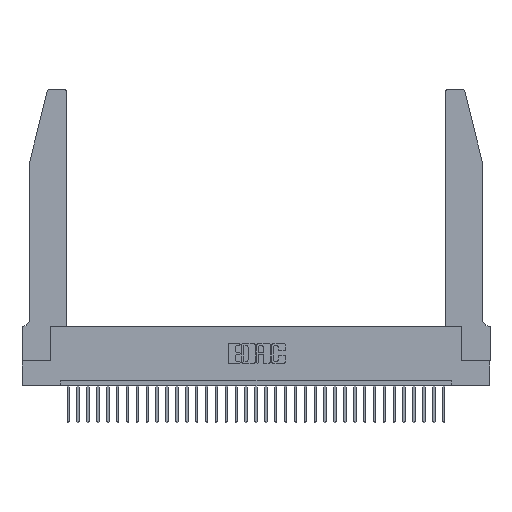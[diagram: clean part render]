
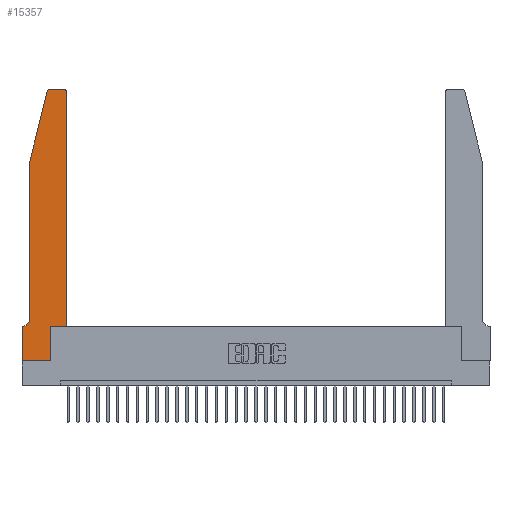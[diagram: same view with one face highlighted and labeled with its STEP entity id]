
A CAD part, top view. The second image highlights one B-rep face of the part: STEP entity #15357.
In plain terms, the highlighted planar face has unit normal (0, 0, 1).
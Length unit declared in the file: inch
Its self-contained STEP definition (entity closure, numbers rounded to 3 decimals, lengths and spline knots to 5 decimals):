
#844 = CARTESIAN_POINT ( 'NONE',  ( 0.0755, 0.42, 0.37 ) ) ;
#1796 = DIRECTION ( 'NONE',  ( -0.239, -0.971, 0. ) ) ;
#1856 = CARTESIAN_POINT ( 'NONE',  ( 0., 0.35, 0.37 ) ) ;
#1897 = ORIENTED_EDGE ( 'NONE', *, *, #27812, .T. ) ;
#1990 = DIRECTION ( 'NONE',  ( 1., 0., 0. ) ) ;
#2243 = EDGE_CURVE ( 'NONE', #21953, #29649, #5907, .T. ) ;
#2429 = LINE ( 'NONE', #12563, #29911 ) ;
#2509 = VERTEX_POINT ( 'NONE', #20249 ) ;
#2885 = CARTESIAN_POINT ( 'NONE',  ( 0., 0., 0.37 ) ) ;
#3509 = DIRECTION ( 'NONE',  ( 1., 0., 0. ) ) ;
#3800 = VECTOR ( 'NONE', #12660, 39.37008 ) ;
#3824 = VERTEX_POINT ( 'NONE', #31055 ) ;
#3830 = ORIENTED_EDGE ( 'NONE', *, *, #16353, .T. ) ;
#4222 = LINE ( 'NONE', #16829, #23867 ) ;
#4612 = AXIS2_PLACEMENT_3D ( 'NONE', #13760, #29898, #32362 ) ;
#4707 = CARTESIAN_POINT ( 'NONE',  ( 0.2865, 0., 0.37 ) ) ;
#4826 = CARTESIAN_POINT ( 'NONE',  ( 0.4505, 2.72, 0.37 ) ) ;
#4992 = EDGE_CURVE ( 'NONE', #17499, #3824, #20780, .T. ) ;
#5145 = EDGE_CURVE ( 'NONE', #8840, #14977, #25309, .T. ) ;
#5199 = LINE ( 'NONE', #14742, #25216 ) ;
#5727 = CARTESIAN_POINT ( 'NONE',  ( 0.0055, 0.35, 0.37 ) ) ;
#5907 = LINE ( 'NONE', #14757, #10103 ) ;
#6216 = LINE ( 'NONE', #22198, #16663 ) ;
#6361 = AXIS2_PLACEMENT_3D ( 'NONE', #10752, #32404, #3509 ) ;
#7086 = EDGE_CURVE ( 'NONE', #14977, #27665, #5199, .T. ) ;
#7990 = LINE ( 'NONE', #28600, #3800 ) ;
#8084 = VERTEX_POINT ( 'NONE', #11076 ) ;
#8706 = CARTESIAN_POINT ( 'NONE',  ( 0.4505, 0.35, 0.37 ) ) ;
#8825 = LINE ( 'NONE', #8706, #29298 ) ;
#8840 = VERTEX_POINT ( 'NONE', #844 ) ;
#9392 = CARTESIAN_POINT ( 'NONE',  ( 0., 0.35, 0.37 ) ) ;
#9546 = PLANE ( 'NONE',  #27710 ) ;
#9677 = VECTOR ( 'NONE', #21092, 39.37008 ) ;
#10103 = VECTOR ( 'NONE', #20571, 39.37008 ) ;
#10752 = CARTESIAN_POINT ( 'NONE',  ( 0.4205, 2.72, 0.37 ) ) ;
#11076 = CARTESIAN_POINT ( 'NONE',  ( 0.284, 2.75, 0.37 ) ) ;
#11282 = DIRECTION ( 'NONE',  ( -1., 0., 0. ) ) ;
#12498 = DIRECTION ( 'NONE',  ( 0., 0., 1. ) ) ;
#12563 = CARTESIAN_POINT ( 'NONE',  ( 0.0755, 2., 0.37 ) ) ;
#12660 = DIRECTION ( 'NONE',  ( 0., 1., 0. ) ) ;
#12894 = ORIENTED_EDGE ( 'NONE', *, *, #18721, .T. ) ;
#13230 = ORIENTED_EDGE ( 'NONE', *, *, #7086, .T. ) ;
#13278 = CARTESIAN_POINT ( 'NONE',  ( 0.0755, 2., 0.37 ) ) ;
#13283 = CARTESIAN_POINT ( 'NONE',  ( 0.2865, 0.35, 0.37 ) ) ;
#13760 = CARTESIAN_POINT ( 'NONE',  ( 0.0055, 0.42, 0.37 ) ) ;
#14742 = CARTESIAN_POINT ( 'NONE',  ( 0.0755, 0.35, 0.37 ) ) ;
#14757 = CARTESIAN_POINT ( 'NONE',  ( 0.2865, 0.35, 0.37 ) ) ;
#14977 = VERTEX_POINT ( 'NONE', #5727 ) ;
#15214 = DIRECTION ( 'NONE',  ( 1., 0., 0. ) ) ;
#15349 = DIRECTION ( 'NONE',  ( 0., 0., 1. ) ) ;
#15357 = ADVANCED_FACE ( 'NONE', ( #33841 ), #9546, .T. ) ;
#15598 = EDGE_CURVE ( 'NONE', #32887, #17499, #7990, .T. ) ;
#16353 = EDGE_CURVE ( 'NONE', #3824, #8084, #4222, .T. ) ;
#16417 = EDGE_CURVE ( 'NONE', #27665, #2509, #17138, .T. ) ;
#16544 = DIRECTION ( 'NONE',  ( 0., -1., 0. ) ) ;
#16663 = VECTOR ( 'NONE', #27501, 39.37008 ) ;
#16829 = CARTESIAN_POINT ( 'NONE',  ( 0.2605, 2.75, 0.37 ) ) ;
#17138 = LINE ( 'NONE', #2885, #32522 ) ;
#17292 = EDGE_CURVE ( 'NONE', #2509, #21953, #6216, .T. ) ;
#17499 = VERTEX_POINT ( 'NONE', #4826 ) ;
#17609 = CARTESIAN_POINT ( 'NONE',  ( 0.0755, 2., 0.37 ) ) ;
#17727 = EDGE_CURVE ( 'NONE', #18711, #19141, #2429, .T. ) ;
#18711 = VERTEX_POINT ( 'NONE', #28447 ) ;
#18721 = EDGE_CURVE ( 'NONE', #8084, #18711, #22405, .T. ) ;
#19141 = VERTEX_POINT ( 'NONE', #17609 ) ;
#20249 = CARTESIAN_POINT ( 'NONE',  ( 0., 0., 0.37 ) ) ;
#20571 = DIRECTION ( 'NONE',  ( 0., 1., 0. ) ) ;
#20780 = CIRCLE ( 'NONE', #6361, 0.03 ) ;
#21092 = DIRECTION ( 'NONE',  ( 0., -1., 0. ) ) ;
#21208 = ORIENTED_EDGE ( 'NONE', *, *, #2243, .T. ) ;
#21593 = DIRECTION ( 'NONE',  ( 1., 0., 0. ) ) ;
#21715 = ORIENTED_EDGE ( 'NONE', *, *, #16417, .T. ) ;
#21953 = VERTEX_POINT ( 'NONE', #4707 ) ;
#22198 = CARTESIAN_POINT ( 'NONE',  ( 0., 0., 0.37 ) ) ;
#22295 = EDGE_LOOP ( 'NONE', ( #3830, #12894, #25731, #1897, #23103, #13230, #21715, #22869, #21208, #25739, #30368, #24260 ) ) ;
#22405 = CIRCLE ( 'NONE', #27373, 0.03 ) ;
#22869 = ORIENTED_EDGE ( 'NONE', *, *, #17292, .T. ) ;
#23103 = ORIENTED_EDGE ( 'NONE', *, *, #5145, .T. ) ;
#23867 = VECTOR ( 'NONE', #11282, 39.37008 ) ;
#24260 = ORIENTED_EDGE ( 'NONE', *, *, #4992, .T. ) ;
#25216 = VECTOR ( 'NONE', #31242, 39.37008 ) ;
#25309 = CIRCLE ( 'NONE', #4612, 0.07 ) ;
#25580 = LINE ( 'NONE', #13278, #9677 ) ;
#25731 = ORIENTED_EDGE ( 'NONE', *, *, #17727, .T. ) ;
#25739 = ORIENTED_EDGE ( 'NONE', *, *, #34164, .T. ) ;
#27373 = AXIS2_PLACEMENT_3D ( 'NONE', #31267, #15349, #1990 ) ;
#27501 = DIRECTION ( 'NONE',  ( 1., 0., 0. ) ) ;
#27665 = VERTEX_POINT ( 'NONE', #9392 ) ;
#27710 = AXIS2_PLACEMENT_3D ( 'NONE', #1856, #12498, #15214 ) ;
#27812 = EDGE_CURVE ( 'NONE', #19141, #8840, #25580, .T. ) ;
#28447 = CARTESIAN_POINT ( 'NONE',  ( 0.25487, 2.72718, 0.37 ) ) ;
#28600 = CARTESIAN_POINT ( 'NONE',  ( 0.4505, 0.35, 0.37 ) ) ;
#29298 = VECTOR ( 'NONE', #21593, 39.37008 ) ;
#29649 = VERTEX_POINT ( 'NONE', #13283 ) ;
#29898 = DIRECTION ( 'NONE',  ( 0., 0., -1. ) ) ;
#29911 = VECTOR ( 'NONE', #1796, 39.37008 ) ;
#30368 = ORIENTED_EDGE ( 'NONE', *, *, #15598, .T. ) ;
#31055 = CARTESIAN_POINT ( 'NONE',  ( 0.4205, 2.75, 0.37 ) ) ;
#31242 = DIRECTION ( 'NONE',  ( -1., 0., 0. ) ) ;
#31267 = CARTESIAN_POINT ( 'NONE',  ( 0.284, 2.72, 0.37 ) ) ;
#31954 = CARTESIAN_POINT ( 'NONE',  ( 0.4505, 0.35, 0.37 ) ) ;
#32362 = DIRECTION ( 'NONE',  ( -1., 0., 0. ) ) ;
#32404 = DIRECTION ( 'NONE',  ( 0., 0., 1. ) ) ;
#32522 = VECTOR ( 'NONE', #16544, 39.37008 ) ;
#32887 = VERTEX_POINT ( 'NONE', #31954 ) ;
#33841 = FACE_OUTER_BOUND ( 'NONE', #22295, .T. ) ;
#34164 = EDGE_CURVE ( 'NONE', #29649, #32887, #8825, .T. ) ;
